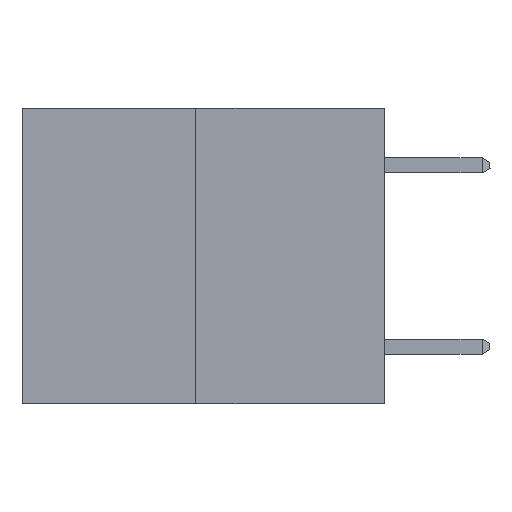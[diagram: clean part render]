
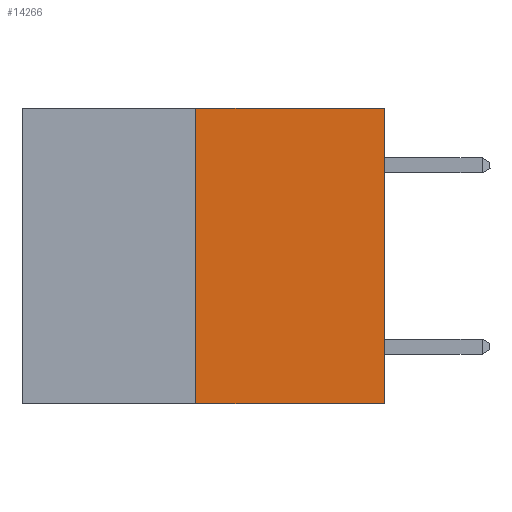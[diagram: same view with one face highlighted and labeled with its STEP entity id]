
A CAD part, left-side view. The second image highlights one B-rep face of the part: STEP entity #14266.
In plain terms, the highlighted planar face has unit normal (-1, 0, 0).
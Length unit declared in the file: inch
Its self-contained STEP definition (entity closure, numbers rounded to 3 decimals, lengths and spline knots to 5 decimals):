
#197 = LINE ( 'NONE', #20537, #24076 ) ;
#559 = EDGE_CURVE ( 'NONE', #11576, #7539, #197, .T. ) ;
#1518 = CARTESIAN_POINT ( 'NONE',  ( 0., 0., 0. ) ) ;
#3093 = VERTEX_POINT ( 'NONE', #1518 ) ;
#3818 = CARTESIAN_POINT ( 'NONE',  ( 0., 0.312, 0. ) ) ;
#3862 = EDGE_LOOP ( 'NONE', ( #12259, #6192, #22594, #23478 ) ) ;
#4178 = PLANE ( 'NONE',  #17714 ) ;
#5743 = VECTOR ( 'NONE', #23406, 39.37008 ) ;
#6192 = ORIENTED_EDGE ( 'NONE', *, *, #559, .T. ) ;
#6619 = LINE ( 'NONE', #7748, #11724 ) ;
#7539 = VERTEX_POINT ( 'NONE', #22635 ) ;
#7748 = CARTESIAN_POINT ( 'NONE',  ( 0., 0.6, 0. ) ) ;
#8445 = DIRECTION ( 'NONE',  ( 0., 0., -1. ) ) ;
#8767 = LINE ( 'NONE', #19154, #5743 ) ;
#8946 = FACE_OUTER_BOUND ( 'NONE', #3862, .T. ) ;
#9901 = DIRECTION ( 'NONE',  ( 0., -1., 0. ) ) ;
#11576 = VERTEX_POINT ( 'NONE', #26900 ) ;
#11724 = VECTOR ( 'NONE', #9901, 39.37008 ) ;
#12259 = ORIENTED_EDGE ( 'NONE', *, *, #15586, .F. ) ;
#12972 = VECTOR ( 'NONE', #13497, 39.37008 ) ;
#13396 = CARTESIAN_POINT ( 'NONE',  ( 0., 0.312, -0.49 ) ) ;
#13497 = DIRECTION ( 'NONE',  ( 0., 0., 1. ) ) ;
#13799 = EDGE_CURVE ( 'NONE', #26326, #3093, #6619, .T. ) ;
#14266 = ADVANCED_FACE ( 'NONE', ( #8946 ), #4178, .F. ) ;
#15028 = DIRECTION ( 'NONE',  ( 1., 0., 0. ) ) ;
#15586 = EDGE_CURVE ( 'NONE', #11576, #26326, #27715, .T. ) ;
#17645 = EDGE_CURVE ( 'NONE', #7539, #3093, #8767, .T. ) ;
#17714 = AXIS2_PLACEMENT_3D ( 'NONE', #25949, #15028, #8445 ) ;
#19154 = CARTESIAN_POINT ( 'NONE',  ( 0., 0., 0. ) ) ;
#20537 = CARTESIAN_POINT ( 'NONE',  ( 0., 0.6, -0.49 ) ) ;
#22594 = ORIENTED_EDGE ( 'NONE', *, *, #17645, .T. ) ;
#22635 = CARTESIAN_POINT ( 'NONE',  ( 0., 0., -0.49 ) ) ;
#22764 = DIRECTION ( 'NONE',  ( 0., -1., 0. ) ) ;
#23406 = DIRECTION ( 'NONE',  ( 0., 0., 1. ) ) ;
#23478 = ORIENTED_EDGE ( 'NONE', *, *, #13799, .F. ) ;
#24076 = VECTOR ( 'NONE', #22764, 39.37008 ) ;
#25949 = CARTESIAN_POINT ( 'NONE',  ( 0., 0.6, 0. ) ) ;
#26326 = VERTEX_POINT ( 'NONE', #3818 ) ;
#26900 = CARTESIAN_POINT ( 'NONE',  ( 0., 0.312, -0.49 ) ) ;
#27715 = LINE ( 'NONE', #13396, #12972 ) ;
